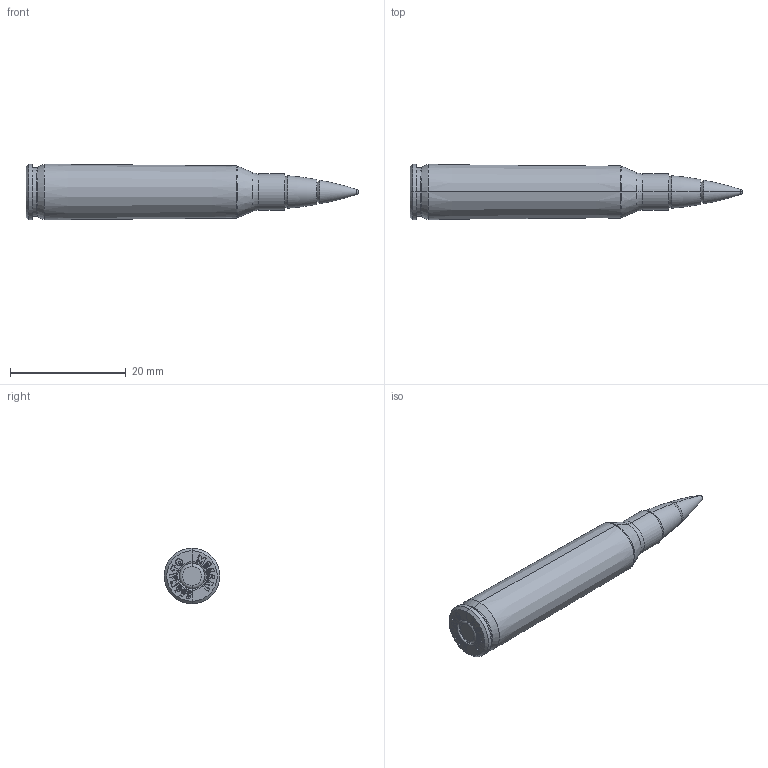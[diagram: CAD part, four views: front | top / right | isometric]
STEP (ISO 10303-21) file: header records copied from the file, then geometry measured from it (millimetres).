
FILE_DESCRIPTION (( 'STEP AP214' ), '1' );
FILE_NAME ('M855A1 62 gr.STEP', '2025-05-18T10:37:42', ( '' ), ( '' ), 'SwSTEP 2.0', 'SolidWorks 2024', '' );
FILE_SCHEMA (( 'AUTOMOTIVE_DESIGN' ));
Length unit declared in the file: millimetre
Products named in the file (1): M855A1 62 gr
Bounding box: 57.39 x 9.6 x 9.6 mm (x, y, z)
Surface area: 1700.2 mm2 (no closed solid volume)
Topology: 0 solids, 5 shells, 369 faces, 1133 edges, 734 vertices
Faces by surface type: bspline 221, plane 96, torus 22, cone 20, cylinder 10
Entity records: 35884 total; most frequent: CARTESIAN_POINT 28195, ORIENTED_EDGE 1870, EDGE_CURVE 1133, DIRECTION 757, B_SPLINE_CURVE_WITH_KNOTS 754, VERTEX_POINT 734, EDGE_LOOP 388, FACE_OUTER_BOUND 369
